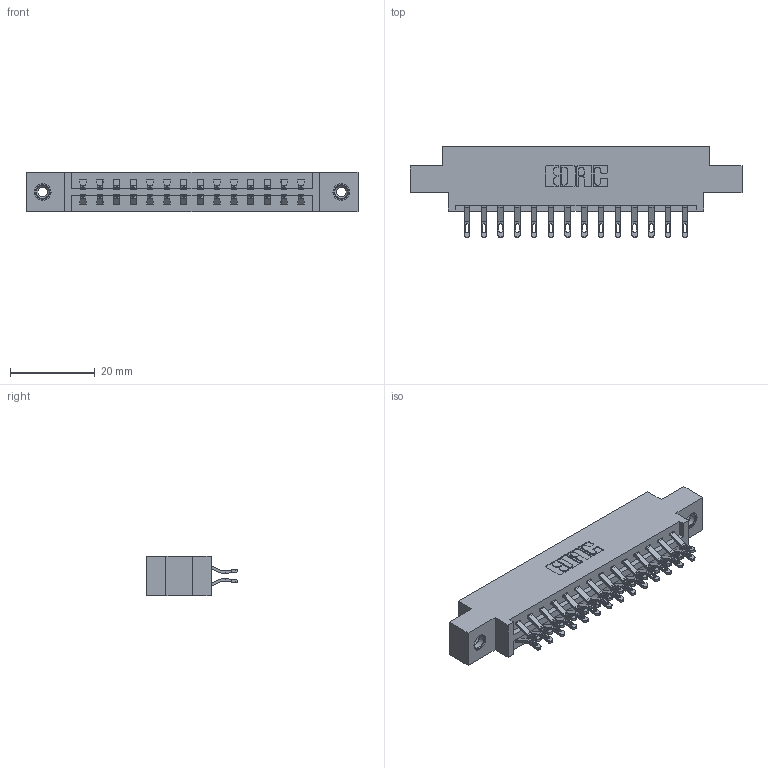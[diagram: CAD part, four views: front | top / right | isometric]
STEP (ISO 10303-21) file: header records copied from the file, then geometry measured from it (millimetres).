
FILE_DESCRIPTION (( 'STEP AP203' ), '1' );
FILE_NAME ('387-028-555-808.STEP', '2018-09-16T23:04:53', ( '' ), ( '' ), 'SwSTEP 2.0', 'SolidWorks 2016', '' );
FILE_SCHEMA (( 'CONFIG_CONTROL_DESIGN' ));
Length unit declared in the file: inch
Products named in the file (4): 387-028-555-808; 337 Part_0.170 Offset - 0.156 Dia-TI; 345-292-001_555 Tail; 345-250-001_345-250-003-102
Assembly tree (31 placements, depth 2):
  387-028-555-808
    337 Part_0.170 Offset - 0.156 Dia-TI
    345-292-001_555 Tail  x28
    345-250-001_345-250-003-102  x2
Bounding box: 78.49 x 21.47 x 9.4 mm (x, y, z)
Volume: 7856 mm3; surface area: 9047 mm2
Topology: 31 solids, 31 shells, 1858 faces, 5751 edges, 3826 vertices
Faces by surface type: plane 1114, cylinder 728, cone 12, torus 4
Entity records: 16120 total; most frequent: CARTESIAN_POINT 2755, ORIENTED_EDGE 2654, DIRECTION 2397, EDGE_CURVE 1327, LINE 1159, VECTOR 1159, VERTEX_POINT 880, AXIS2_PLACEMENT_3D 619
